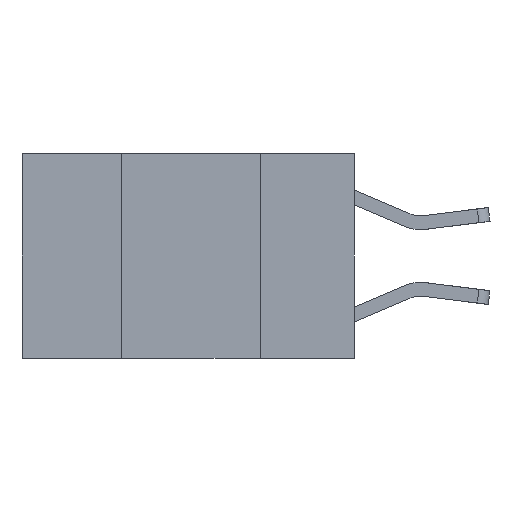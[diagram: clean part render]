
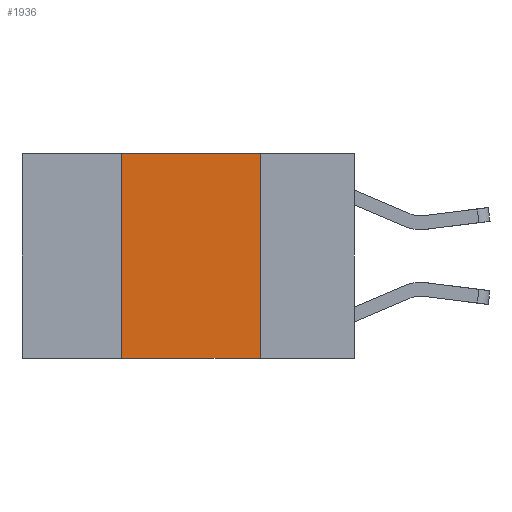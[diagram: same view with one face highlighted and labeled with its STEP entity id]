
A CAD part, left-side view. The second image highlights one B-rep face of the part: STEP entity #1936.
In plain terms, the highlighted planar face has unit normal (-1, 0, 0).
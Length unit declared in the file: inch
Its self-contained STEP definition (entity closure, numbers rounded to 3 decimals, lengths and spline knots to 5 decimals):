
#520 = CARTESIAN_POINT ( 'NONE',  ( 0., 0.6, 0. ) ) ;
#1435 = DIRECTION ( 'NONE',  ( 0., -1., 0. ) ) ;
#1547 = VERTEX_POINT ( 'NONE', #11563 ) ;
#1835 = EDGE_LOOP ( 'NONE', ( #6916, #9522, #11032, #7340 ) ) ;
#1936 = ADVANCED_FACE ( 'NONE', ( #6350 ), #8512, .F. ) ;
#2455 = EDGE_CURVE ( 'NONE', #9512, #12419, #10637, .T. ) ;
#3151 = VERTEX_POINT ( 'NONE', #5746 ) ;
#4585 = CARTESIAN_POINT ( 'NONE',  ( 0., 0.42, 0. ) ) ;
#5051 = DIRECTION ( 'NONE',  ( 0., -1., 0. ) ) ;
#5611 = DIRECTION ( 'NONE',  ( 0., 0., -1. ) ) ;
#5746 = CARTESIAN_POINT ( 'NONE',  ( 0., 0.17, -0.37 ) ) ;
#6029 = CARTESIAN_POINT ( 'NONE',  ( 0., 0.42, 0. ) ) ;
#6181 = EDGE_CURVE ( 'NONE', #12419, #3151, #11428, .T. ) ;
#6288 = VECTOR ( 'NONE', #10592, 39.37008 ) ;
#6350 = FACE_OUTER_BOUND ( 'NONE', #1835, .T. ) ;
#6391 = EDGE_CURVE ( 'NONE', #1547, #9512, #7070, .T. ) ;
#6407 = EDGE_CURVE ( 'NONE', #1547, #3151, #11569, .T. ) ;
#6436 = VECTOR ( 'NONE', #5051, 39.37008 ) ;
#6753 = VECTOR ( 'NONE', #11802, 39.37008 ) ;
#6916 = ORIENTED_EDGE ( 'NONE', *, *, #6181, .F. ) ;
#7070 = LINE ( 'NONE', #6029, #6753 ) ;
#7340 = ORIENTED_EDGE ( 'NONE', *, *, #6407, .T. ) ;
#8512 = PLANE ( 'NONE',  #12164 ) ;
#9512 = VERTEX_POINT ( 'NONE', #4585 ) ;
#9522 = ORIENTED_EDGE ( 'NONE', *, *, #2455, .F. ) ;
#9950 = CARTESIAN_POINT ( 'NONE',  ( 0., 0.6, -0.37 ) ) ;
#10336 = CARTESIAN_POINT ( 'NONE',  ( 0., 0.6, 0. ) ) ;
#10592 = DIRECTION ( 'NONE',  ( 0., 0., -1. ) ) ;
#10637 = LINE ( 'NONE', #10336, #12217 ) ;
#11032 = ORIENTED_EDGE ( 'NONE', *, *, #6391, .F. ) ;
#11428 = LINE ( 'NONE', #11529, #6288 ) ;
#11434 = DIRECTION ( 'NONE',  ( 1., 0., 0. ) ) ;
#11436 = CARTESIAN_POINT ( 'NONE',  ( 0., 0.17, 0. ) ) ;
#11529 = CARTESIAN_POINT ( 'NONE',  ( 0., 0.17, 0. ) ) ;
#11563 = CARTESIAN_POINT ( 'NONE',  ( 0., 0.42, -0.37 ) ) ;
#11569 = LINE ( 'NONE', #9950, #6436 ) ;
#11802 = DIRECTION ( 'NONE',  ( 0., 0., 1. ) ) ;
#12164 = AXIS2_PLACEMENT_3D ( 'NONE', #520, #11434, #5611 ) ;
#12217 = VECTOR ( 'NONE', #1435, 39.37008 ) ;
#12419 = VERTEX_POINT ( 'NONE', #11436 ) ;
